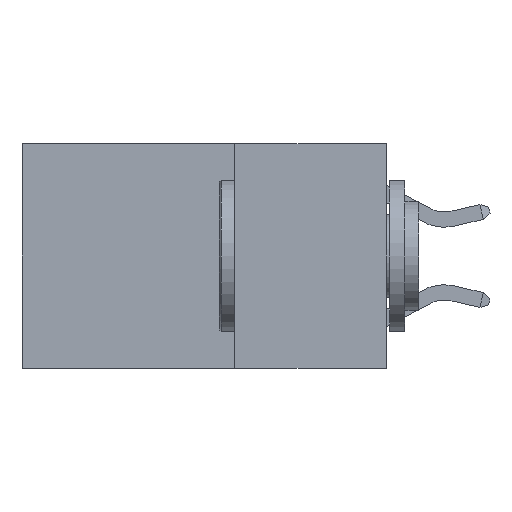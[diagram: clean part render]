
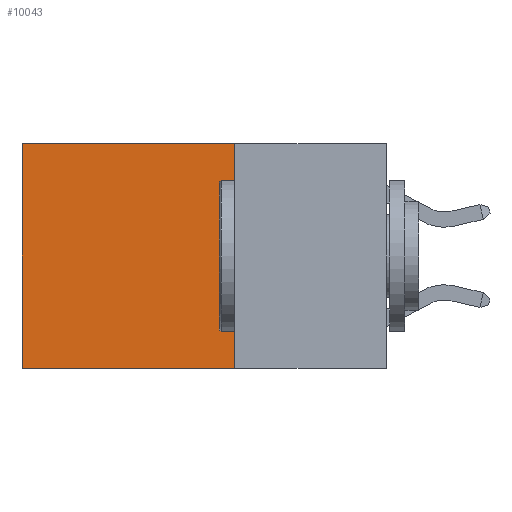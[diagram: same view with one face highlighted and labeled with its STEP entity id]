
A CAD part, left-side view. The second image highlights one B-rep face of the part: STEP entity #10043.
In plain terms, the highlighted planar face has unit normal (-1, 0, 0).
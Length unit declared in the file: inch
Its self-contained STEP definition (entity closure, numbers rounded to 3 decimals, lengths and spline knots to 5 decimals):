
#273 = VERTEX_POINT ( 'NONE', #8675 ) ;
#445 = CARTESIAN_POINT ( 'NONE',  ( 0.2625, 0.25, 0. ) ) ;
#508 = ORIENTED_EDGE ( 'NONE', *, *, #4370, .T. ) ;
#1272 = VERTEX_POINT ( 'NONE', #3239 ) ;
#1772 = EDGE_CURVE ( 'NONE', #10674, #9590, #9610, .T. ) ;
#2514 = EDGE_LOOP ( 'NONE', ( #508, #11263, #5606, #12292 ) ) ;
#3239 = CARTESIAN_POINT ( 'NONE',  ( 0.2625, 0.6, 0. ) ) ;
#3438 = DIRECTION ( 'NONE',  ( 0., 0., -1. ) ) ;
#3569 = LINE ( 'NONE', #6276, #10682 ) ;
#4304 = DIRECTION ( 'NONE',  ( 0., 1., 0. ) ) ;
#4370 = EDGE_CURVE ( 'NONE', #1272, #9590, #10899, .T. ) ;
#4748 = LINE ( 'NONE', #445, #7076 ) ;
#4957 = CARTESIAN_POINT ( 'NONE',  ( 0.2625, 0.25, -0.37 ) ) ;
#5072 = DIRECTION ( 'NONE',  ( 0., 1., 0. ) ) ;
#5333 = CARTESIAN_POINT ( 'NONE',  ( 0.2625, 0.6, -0.37 ) ) ;
#5606 = ORIENTED_EDGE ( 'NONE', *, *, #9619, .F. ) ;
#5670 = DIRECTION ( 'NONE',  ( 1., 0., 0. ) ) ;
#6276 = CARTESIAN_POINT ( 'NONE',  ( 0.2625, 0.25, 0. ) ) ;
#6575 = CARTESIAN_POINT ( 'NONE',  ( 0.2625, 0.25, -0.37 ) ) ;
#6635 = PLANE ( 'NONE',  #9984 ) ;
#6749 = VECTOR ( 'NONE', #5072, 39.37008 ) ;
#7076 = VECTOR ( 'NONE', #4304, 39.37008 ) ;
#7617 = CARTESIAN_POINT ( 'NONE',  ( 0.2625, 0.25, 0. ) ) ;
#8675 = CARTESIAN_POINT ( 'NONE',  ( 0.2625, 0.25, 0. ) ) ;
#9590 = VERTEX_POINT ( 'NONE', #5333 ) ;
#9610 = LINE ( 'NONE', #4957, #6749 ) ;
#9619 = EDGE_CURVE ( 'NONE', #273, #10674, #3569, .T. ) ;
#9984 = AXIS2_PLACEMENT_3D ( 'NONE', #7617, #5670, #12368 ) ;
#10043 = ADVANCED_FACE ( 'NONE', ( #10961 ), #6635, .F. ) ;
#10268 = DIRECTION ( 'NONE',  ( 0., 0., -1. ) ) ;
#10436 = EDGE_CURVE ( 'NONE', #273, #1272, #4748, .T. ) ;
#10611 = VECTOR ( 'NONE', #10268, 39.37008 ) ;
#10674 = VERTEX_POINT ( 'NONE', #6575 ) ;
#10682 = VECTOR ( 'NONE', #3438, 39.37008 ) ;
#10899 = LINE ( 'NONE', #12126, #10611 ) ;
#10961 = FACE_OUTER_BOUND ( 'NONE', #2514, .T. ) ;
#11263 = ORIENTED_EDGE ( 'NONE', *, *, #1772, .F. ) ;
#12126 = CARTESIAN_POINT ( 'NONE',  ( 0.2625, 0.6, 0. ) ) ;
#12292 = ORIENTED_EDGE ( 'NONE', *, *, #10436, .T. ) ;
#12368 = DIRECTION ( 'NONE',  ( 0., 0., -1. ) ) ;
